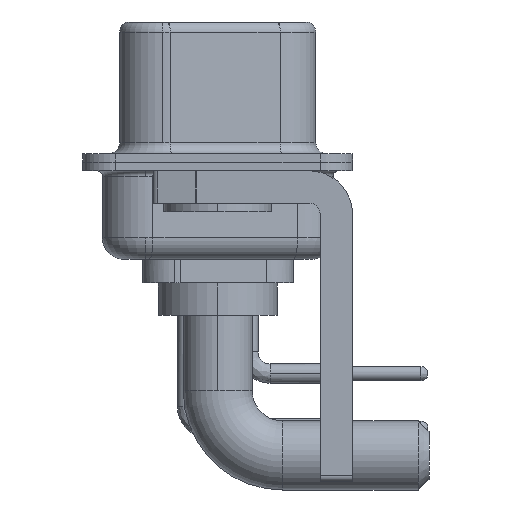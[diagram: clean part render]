
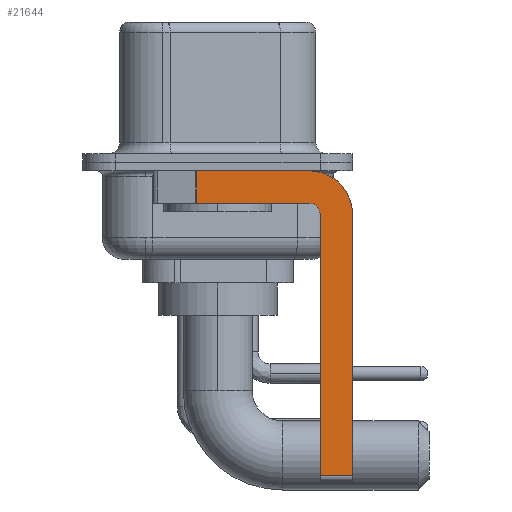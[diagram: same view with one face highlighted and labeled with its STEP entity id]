
A CAD part, left-side view. The second image highlights one B-rep face of the part: STEP entity #21644.
In plain terms, the highlighted planar face has unit normal (-1, 0, 0).
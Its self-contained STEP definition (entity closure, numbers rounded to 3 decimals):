
#295 = AXIS2_PLACEMENT_3D ( 'NONE', #17476, #8487, #8218 ) ;
#962 = CARTESIAN_POINT ( 'NONE',  ( -2.9, 3., -0.4 ) ) ;
#1058 = CARTESIAN_POINT ( 'NONE',  ( -2.9, -4.25, -0.4 ) ) ;
#1218 = EDGE_CURVE ( 'NONE', #7795, #19072, #22820, .T. ) ;
#1347 = DIRECTION ( 'NONE',  ( 0., -1., 0. ) ) ;
#1442 = CARTESIAN_POINT ( 'NONE',  ( -2.9, -6.25, -14.55 ) ) ;
#1773 = CARTESIAN_POINT ( 'NONE',  ( -2.9, 0.978, -1.9 ) ) ;
#1971 = DIRECTION ( 'NONE',  ( 0., 0., -1. ) ) ;
#2146 = ORIENTED_EDGE ( 'NONE', *, *, #9610, .F. ) ;
#2296 = CARTESIAN_POINT ( 'NONE',  ( -2.9, -4.25, -2.4 ) ) ;
#2377 = VERTEX_POINT ( 'NONE', #18014 ) ;
#2869 = LINE ( 'NONE', #24622, #26697 ) ;
#3253 = CARTESIAN_POINT ( 'NONE',  ( -2.9, 0.978, -1.9 ) ) ;
#3821 = EDGE_CURVE ( 'NONE', #9307, #19072, #25119, .T. ) ;
#3927 = VECTOR ( 'NONE', #16168, 1000. ) ;
#4362 = EDGE_CURVE ( 'NONE', #6080, #7795, #18765, .T. ) ;
#5829 = CARTESIAN_POINT ( 'NONE',  ( -2.9, -4.75, -14.8 ) ) ;
#6080 = VERTEX_POINT ( 'NONE', #1058 ) ;
#6288 = ORIENTED_EDGE ( 'NONE', *, *, #12190, .F. ) ;
#6539 = EDGE_CURVE ( 'NONE', #9307, #13601, #25548, .T. ) ;
#7102 = VERTEX_POINT ( 'NONE', #26492 ) ;
#7653 = ORIENTED_EDGE ( 'NONE', *, *, #3821, .T. ) ;
#7795 = VERTEX_POINT ( 'NONE', #21483 ) ;
#8218 = DIRECTION ( 'NONE',  ( 0., 0., -1. ) ) ;
#8487 = DIRECTION ( 'NONE',  ( 1., 0., 0. ) ) ;
#9307 = VERTEX_POINT ( 'NONE', #22339 ) ;
#9610 = EDGE_CURVE ( 'NONE', #2377, #6080, #11970, .T. ) ;
#10036 = EDGE_CURVE ( 'NONE', #2377, #14053, #23226, .T. ) ;
#10653 = ORIENTED_EDGE ( 'NONE', *, *, #1218, .F. ) ;
#11580 = ORIENTED_EDGE ( 'NONE', *, *, #6539, .F. ) ;
#11970 = LINE ( 'NONE', #962, #17505 ) ;
#12190 = EDGE_CURVE ( 'NONE', #13601, #7102, #25838, .T. ) ;
#12553 = PLANE ( 'NONE',  #295 ) ;
#12867 = ORIENTED_EDGE ( 'NONE', *, *, #10036, .T. ) ;
#13323 = AXIS2_PLACEMENT_3D ( 'NONE', #2296, #13865, #13713 ) ;
#13601 = VERTEX_POINT ( 'NONE', #23230 ) ;
#13713 = DIRECTION ( 'NONE',  ( 0., 0., 1. ) ) ;
#13721 = VECTOR ( 'NONE', #18690, 1000. ) ;
#13865 = DIRECTION ( 'NONE',  ( -1., 0., 0. ) ) ;
#14053 = VERTEX_POINT ( 'NONE', #1773 ) ;
#16043 = ORIENTED_EDGE ( 'NONE', *, *, #4362, .F. ) ;
#16168 = DIRECTION ( 'NONE',  ( 0., 0., -1. ) ) ;
#16819 = CARTESIAN_POINT ( 'NONE',  ( -2.9, -4.25, -14.55 ) ) ;
#17476 = CARTESIAN_POINT ( 'NONE',  ( -2.9, -4.25, -2.4 ) ) ;
#17505 = VECTOR ( 'NONE', #22580, 1000. ) ;
#17869 = ORIENTED_EDGE ( 'NONE', *, *, #21401, .F. ) ;
#18014 = CARTESIAN_POINT ( 'NONE',  ( -2.9, 0.978, -0.4 ) ) ;
#18311 = AXIS2_PLACEMENT_3D ( 'NONE', #24156, #19501, #1971 ) ;
#18690 = DIRECTION ( 'NONE',  ( 0., 0., 1. ) ) ;
#18765 = CIRCLE ( 'NONE', #18311, 2. ) ;
#19072 = VERTEX_POINT ( 'NONE', #1442 ) ;
#19171 = DIRECTION ( 'NONE',  ( 0., 0., -1. ) ) ;
#19501 = DIRECTION ( 'NONE',  ( 1., 0., 0. ) ) ;
#19964 = DIRECTION ( 'NONE',  ( 0., 1., 0. ) ) ;
#21401 = EDGE_CURVE ( 'NONE', #7102, #14053, #2869, .T. ) ;
#21483 = CARTESIAN_POINT ( 'NONE',  ( -2.9, -6.25, -2.4 ) ) ;
#21644 = ADVANCED_FACE ( 'NONE', ( #24160 ), #12553, .F. ) ;
#22339 = CARTESIAN_POINT ( 'NONE',  ( -2.9, -4.75, -14.55 ) ) ;
#22580 = DIRECTION ( 'NONE',  ( 0., -1., 0. ) ) ;
#22675 = EDGE_LOOP ( 'NONE', ( #2146, #12867, #17869, #6288, #11580, #7653, #10653, #16043 ) ) ;
#22820 = LINE ( 'NONE', #27481, #3927 ) ;
#23226 = LINE ( 'NONE', #3253, #27732 ) ;
#23230 = CARTESIAN_POINT ( 'NONE',  ( -2.9, -4.75, -2.4 ) ) ;
#24156 = CARTESIAN_POINT ( 'NONE',  ( -2.9, -4.25, -2.4 ) ) ;
#24160 = FACE_OUTER_BOUND ( 'NONE', #22675, .T. ) ;
#24622 = CARTESIAN_POINT ( 'NONE',  ( -2.9, -4.25, -1.9 ) ) ;
#25119 = LINE ( 'NONE', #16819, #26973 ) ;
#25548 = LINE ( 'NONE', #5829, #13721 ) ;
#25838 = CIRCLE ( 'NONE', #13323, 0.5 ) ;
#26492 = CARTESIAN_POINT ( 'NONE',  ( -2.9, -4.25, -1.9 ) ) ;
#26697 = VECTOR ( 'NONE', #19964, 1000. ) ;
#26973 = VECTOR ( 'NONE', #1347, 1000. ) ;
#27481 = CARTESIAN_POINT ( 'NONE',  ( -2.9, -6.25, -2.4 ) ) ;
#27732 = VECTOR ( 'NONE', #19171, 1000. ) ;
